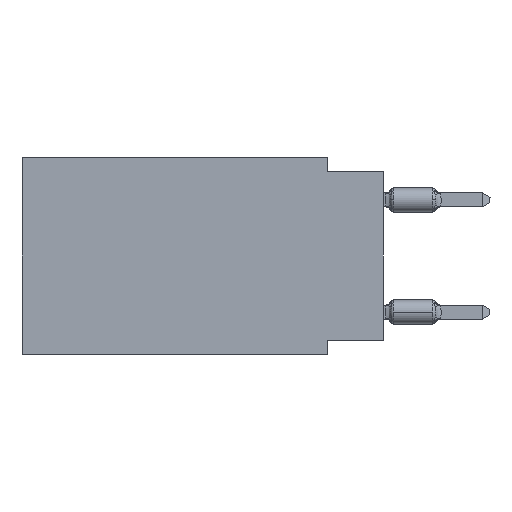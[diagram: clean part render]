
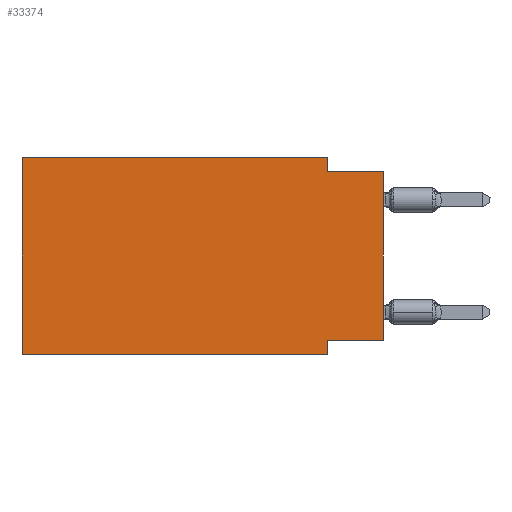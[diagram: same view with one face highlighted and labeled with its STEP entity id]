
A CAD part, left-side view. The second image highlights one B-rep face of the part: STEP entity #33374.
In plain terms, the highlighted planar face has unit normal (-1, 0, 0).
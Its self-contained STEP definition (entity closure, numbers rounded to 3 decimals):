
#4470 = VECTOR ( 'NONE', #38704, 1000. ) ;
#5795 = VERTEX_POINT ( 'NONE', #56635 ) ;
#6322 = FACE_OUTER_BOUND ( 'NONE', #34726, .T. ) ;
#7227 = DIRECTION ( 'NONE',  ( 0., 0., 1. ) ) ;
#9532 = CARTESIAN_POINT ( 'NONE',  ( 0., 2.54, -8.89 ) ) ;
#10474 = EDGE_CURVE ( 'NONE', #11649, #19021, #43001, .T. ) ;
#11416 = VECTOR ( 'NONE', #7227, 1000. ) ;
#11649 = VERTEX_POINT ( 'NONE', #12310 ) ;
#12310 = CARTESIAN_POINT ( 'NONE',  ( 0., 16.383, 0. ) ) ;
#13875 = EDGE_CURVE ( 'NONE', #50780, #33363, #46537, .T. ) ;
#13975 = EDGE_CURVE ( 'NONE', #31057, #11649, #42502, .T. ) ;
#14426 = DIRECTION ( 'NONE',  ( 0., -1., 0. ) ) ;
#14653 = DIRECTION ( 'NONE',  ( 0., 0., -1. ) ) ;
#15902 = LINE ( 'NONE', #38833, #48909 ) ;
#17453 = EDGE_CURVE ( 'NONE', #31057, #18642, #39700, .T. ) ;
#18394 = VECTOR ( 'NONE', #14426, 1000. ) ;
#18642 = VERTEX_POINT ( 'NONE', #37629 ) ;
#18898 = AXIS2_PLACEMENT_3D ( 'NONE', #24691, #41334, #14653 ) ;
#19021 = VERTEX_POINT ( 'NONE', #43607 ) ;
#20095 = CARTESIAN_POINT ( 'NONE',  ( 0., 0., -0.635 ) ) ;
#20136 = VECTOR ( 'NONE', #31890, 1000. ) ;
#20449 = VECTOR ( 'NONE', #21930, 1000. ) ;
#21127 = EDGE_CURVE ( 'NONE', #42250, #18642, #40216, .T. ) ;
#21563 = LINE ( 'NONE', #35338, #26535 ) ;
#21930 = DIRECTION ( 'NONE',  ( 0., 1., 0. ) ) ;
#22022 = EDGE_CURVE ( 'NONE', #50780, #42250, #43462, .T. ) ;
#24691 = CARTESIAN_POINT ( 'NONE',  ( 0., 16.383, 0. ) ) ;
#25007 = DIRECTION ( 'NONE',  ( 0., 0., 1. ) ) ;
#25634 = DIRECTION ( 'NONE',  ( 0., 0., -1. ) ) ;
#26535 = VECTOR ( 'NONE', #35057, 1000. ) ;
#29217 = ORIENTED_EDGE ( 'NONE', *, *, #13875, .T. ) ;
#29904 = ORIENTED_EDGE ( 'NONE', *, *, #10474, .F. ) ;
#31057 = VERTEX_POINT ( 'NONE', #45834 ) ;
#31890 = DIRECTION ( 'NONE',  ( 0., 0., -1. ) ) ;
#31892 = CARTESIAN_POINT ( 'NONE',  ( 0., 2.54, -8.255 ) ) ;
#32806 = ORIENTED_EDGE ( 'NONE', *, *, #21127, .F. ) ;
#32987 = ORIENTED_EDGE ( 'NONE', *, *, #17453, .T. ) ;
#33363 = VERTEX_POINT ( 'NONE', #20095 ) ;
#33374 = ADVANCED_FACE ( 'NONE', ( #6322 ), #50841, .F. ) ;
#34726 = EDGE_LOOP ( 'NONE', ( #29217, #41259, #47866, #29904, #39130, #32987, #32806, #34851 ) ) ;
#34851 = ORIENTED_EDGE ( 'NONE', *, *, #22022, .F. ) ;
#35057 = DIRECTION ( 'NONE',  ( 0., -1., 0. ) ) ;
#35338 = CARTESIAN_POINT ( 'NONE',  ( 0., 0., -0.635 ) ) ;
#37339 = EDGE_CURVE ( 'NONE', #5795, #33363, #21563, .T. ) ;
#37629 = CARTESIAN_POINT ( 'NONE',  ( 0., 2.54, -8.89 ) ) ;
#38704 = DIRECTION ( 'NONE',  ( 0., -1., 0. ) ) ;
#38833 = CARTESIAN_POINT ( 'NONE',  ( 0., 2.54, 0. ) ) ;
#39130 = ORIENTED_EDGE ( 'NONE', *, *, #13975, .F. ) ;
#39700 = LINE ( 'NONE', #48340, #18394 ) ;
#40216 = LINE ( 'NONE', #9532, #20136 ) ;
#41259 = ORIENTED_EDGE ( 'NONE', *, *, #37339, .F. ) ;
#41334 = DIRECTION ( 'NONE',  ( 1., 0., 0. ) ) ;
#42250 = VERTEX_POINT ( 'NONE', #31892 ) ;
#42502 = LINE ( 'NONE', #50875, #48343 ) ;
#43001 = LINE ( 'NONE', #43284, #4470 ) ;
#43284 = CARTESIAN_POINT ( 'NONE',  ( 0., 16.383, 0. ) ) ;
#43462 = LINE ( 'NONE', #43743, #20449 ) ;
#43607 = CARTESIAN_POINT ( 'NONE',  ( 0., 2.54, 0. ) ) ;
#43743 = CARTESIAN_POINT ( 'NONE',  ( 0., 0., -8.255 ) ) ;
#45834 = CARTESIAN_POINT ( 'NONE',  ( 0., 16.383, -8.89 ) ) ;
#46537 = LINE ( 'NONE', #46820, #11416 ) ;
#46820 = CARTESIAN_POINT ( 'NONE',  ( 0., 0., 0. ) ) ;
#47866 = ORIENTED_EDGE ( 'NONE', *, *, #55463, .F. ) ;
#47869 = CARTESIAN_POINT ( 'NONE',  ( 0., 0., -8.255 ) ) ;
#48340 = CARTESIAN_POINT ( 'NONE',  ( 0., 16.383, -8.89 ) ) ;
#48343 = VECTOR ( 'NONE', #25007, 1000. ) ;
#48909 = VECTOR ( 'NONE', #25634, 1000. ) ;
#50780 = VERTEX_POINT ( 'NONE', #47869 ) ;
#50841 = PLANE ( 'NONE',  #18898 ) ;
#50875 = CARTESIAN_POINT ( 'NONE',  ( 0., 16.383, 0. ) ) ;
#55463 = EDGE_CURVE ( 'NONE', #19021, #5795, #15902, .T. ) ;
#56635 = CARTESIAN_POINT ( 'NONE',  ( 0., 2.54, -0.635 ) ) ;
